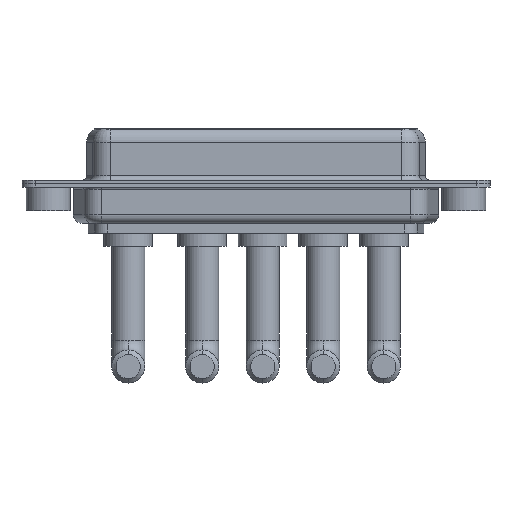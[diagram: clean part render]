
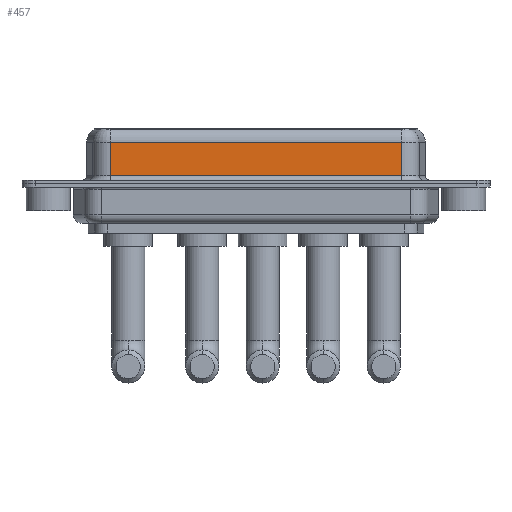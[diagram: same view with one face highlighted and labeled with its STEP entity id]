
A CAD part, front view. The second image highlights one B-rep face of the part: STEP entity #457.
In plain terms, the highlighted planar face has unit normal (0, -1, 0).
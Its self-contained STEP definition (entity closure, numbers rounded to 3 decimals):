
#33 = CARTESIAN_POINT ( 'NONE',  ( 40.037, -3.95, 0.9 ) ) ;
#234 = VECTOR ( 'NONE', #3442, 1000. ) ;
#294 = LINE ( 'NONE', #1192, #10765 ) ;
#457 = ADVANCED_FACE ( 'NONE', ( #11377 ), #5532, .F. ) ;
#1192 = CARTESIAN_POINT ( 'NONE',  ( 40.037, -3.95, 4.65 ) ) ;
#1292 = EDGE_CURVE ( 'NONE', #10344, #5392, #10440, .T. ) ;
#1652 = ORIENTED_EDGE ( 'NONE', *, *, #8143, .T. ) ;
#2391 = CARTESIAN_POINT ( 'NONE',  ( 40.037, -3.95, 6.4 ) ) ;
#2515 = DIRECTION ( 'NONE',  ( 0., 0., 1. ) ) ;
#3442 = DIRECTION ( 'NONE',  ( 1., 0., 0. ) ) ;
#4482 = CARTESIAN_POINT ( 'NONE',  ( 40.037, -3.95, 0.9 ) ) ;
#5119 = DIRECTION ( 'NONE',  ( -1., 0., 0. ) ) ;
#5309 = LINE ( 'NONE', #6206, #12462 ) ;
#5316 = ORIENTED_EDGE ( 'NONE', *, *, #5378, .T. ) ;
#5378 = EDGE_CURVE ( 'NONE', #10054, #7373, #294, .T. ) ;
#5392 = VERTEX_POINT ( 'NONE', #33 ) ;
#5532 = PLANE ( 'NONE',  #8351 ) ;
#6206 = CARTESIAN_POINT ( 'NONE',  ( 40.037, -3.95, 6.4 ) ) ;
#6793 = ORIENTED_EDGE ( 'NONE', *, *, #1292, .T. ) ;
#7373 = VERTEX_POINT ( 'NONE', #11771 ) ;
#7466 = CARTESIAN_POINT ( 'NONE',  ( 7.013, -3.95, 0.9 ) ) ;
#7887 = EDGE_LOOP ( 'NONE', ( #11759, #5316, #1652, #6793 ) ) ;
#8143 = EDGE_CURVE ( 'NONE', #7373, #10344, #8252, .T. ) ;
#8252 = LINE ( 'NONE', #8315, #9963 ) ;
#8315 = CARTESIAN_POINT ( 'NONE',  ( 7.013, -3.95, 6.4 ) ) ;
#8351 = AXIS2_PLACEMENT_3D ( 'NONE', #2391, #9480, #2515 ) ;
#9480 = DIRECTION ( 'NONE',  ( 0., 1., 0. ) ) ;
#9497 = EDGE_CURVE ( 'NONE', #10054, #5392, #5309, .T. ) ;
#9963 = VECTOR ( 'NONE', #12330, 1000. ) ;
#10054 = VERTEX_POINT ( 'NONE', #12081 ) ;
#10344 = VERTEX_POINT ( 'NONE', #7466 ) ;
#10440 = LINE ( 'NONE', #4482, #234 ) ;
#10765 = VECTOR ( 'NONE', #5119, 1000. ) ;
#11377 = FACE_OUTER_BOUND ( 'NONE', #7887, .T. ) ;
#11396 = DIRECTION ( 'NONE',  ( 0., 0., -1. ) ) ;
#11759 = ORIENTED_EDGE ( 'NONE', *, *, #9497, .F. ) ;
#11771 = CARTESIAN_POINT ( 'NONE',  ( 7.013, -3.95, 4.65 ) ) ;
#12081 = CARTESIAN_POINT ( 'NONE',  ( 40.037, -3.95, 4.65 ) ) ;
#12330 = DIRECTION ( 'NONE',  ( 0., 0., -1. ) ) ;
#12462 = VECTOR ( 'NONE', #11396, 1000. ) ;
